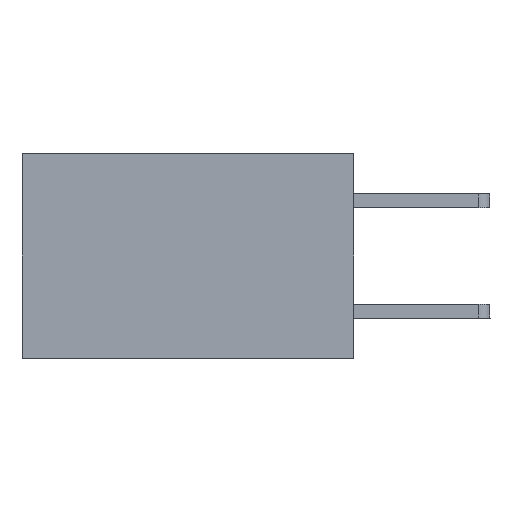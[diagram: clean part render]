
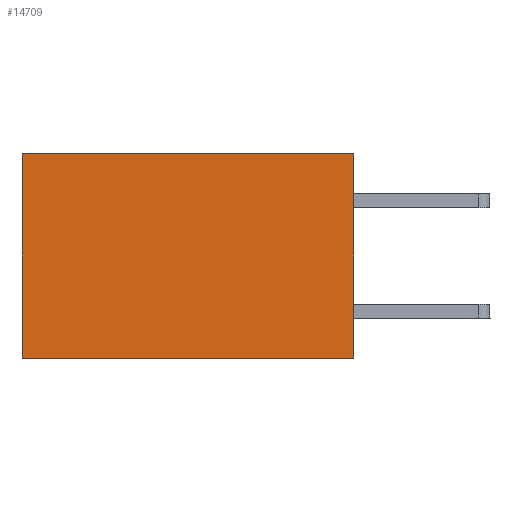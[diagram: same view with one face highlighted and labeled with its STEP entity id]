
A CAD part, left-side view. The second image highlights one B-rep face of the part: STEP entity #14709.
In plain terms, the highlighted planar face has unit normal (-1, 0, 0).
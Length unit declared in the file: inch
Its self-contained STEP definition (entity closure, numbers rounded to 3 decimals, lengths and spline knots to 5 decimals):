
#1321 = CARTESIAN_POINT ( 'NONE',  ( 0.2875, 0., 0. ) ) ;
#1728 = EDGE_CURVE ( 'NONE', #2367, #10280, #5850, .T. ) ;
#1933 = DIRECTION ( 'NONE',  ( 0., 0., -1. ) ) ;
#2138 = LINE ( 'NONE', #5741, #4525 ) ;
#2367 = VERTEX_POINT ( 'NONE', #13669 ) ;
#2877 = VECTOR ( 'NONE', #1933, 39.37008 ) ;
#3353 = DIRECTION ( 'NONE',  ( 0., 1., 0. ) ) ;
#3823 = ORIENTED_EDGE ( 'NONE', *, *, #1728, .F. ) ;
#4215 = LINE ( 'NONE', #5221, #2877 ) ;
#4525 = VECTOR ( 'NONE', #3353, 39.37008 ) ;
#4901 = ORIENTED_EDGE ( 'NONE', *, *, #7709, .T. ) ;
#4930 = PLANE ( 'NONE',  #6812 ) ;
#5221 = CARTESIAN_POINT ( 'NONE',  ( 0.2875, 0.6, 0. ) ) ;
#5741 = CARTESIAN_POINT ( 'NONE',  ( 0.2875, 0., 0. ) ) ;
#5850 = LINE ( 'NONE', #10499, #12642 ) ;
#6453 = CARTESIAN_POINT ( 'NONE',  ( 0.2875, 0., -0.37 ) ) ;
#6812 = AXIS2_PLACEMENT_3D ( 'NONE', #1321, #10638, #8597 ) ;
#6853 = CARTESIAN_POINT ( 'NONE',  ( 0.2875, 0.6, -0.37 ) ) ;
#7210 = EDGE_CURVE ( 'NONE', #11978, #9052, #4215, .T. ) ;
#7233 = EDGE_CURVE ( 'NONE', #10280, #9052, #9878, .T. ) ;
#7252 = EDGE_LOOP ( 'NONE', ( #12729, #7450, #3823, #4901 ) ) ;
#7450 = ORIENTED_EDGE ( 'NONE', *, *, #7233, .F. ) ;
#7600 = DIRECTION ( 'NONE',  ( 0., 1., 0. ) ) ;
#7709 = EDGE_CURVE ( 'NONE', #2367, #11978, #2138, .T. ) ;
#8219 = DIRECTION ( 'NONE',  ( 0., 0., -1. ) ) ;
#8597 = DIRECTION ( 'NONE',  ( 0., 0., -1. ) ) ;
#9052 = VERTEX_POINT ( 'NONE', #6853 ) ;
#9426 = FACE_OUTER_BOUND ( 'NONE', #7252, .T. ) ;
#9721 = VECTOR ( 'NONE', #7600, 39.37008 ) ;
#9878 = LINE ( 'NONE', #6453, #9721 ) ;
#10280 = VERTEX_POINT ( 'NONE', #11043 ) ;
#10499 = CARTESIAN_POINT ( 'NONE',  ( 0.2875, 0., 0. ) ) ;
#10638 = DIRECTION ( 'NONE',  ( 1., 0., 0. ) ) ;
#11043 = CARTESIAN_POINT ( 'NONE',  ( 0.2875, 0., -0.37 ) ) ;
#11978 = VERTEX_POINT ( 'NONE', #12786 ) ;
#12642 = VECTOR ( 'NONE', #8219, 39.37008 ) ;
#12729 = ORIENTED_EDGE ( 'NONE', *, *, #7210, .T. ) ;
#12786 = CARTESIAN_POINT ( 'NONE',  ( 0.2875, 0.6, 0. ) ) ;
#13669 = CARTESIAN_POINT ( 'NONE',  ( 0.2875, 0., 0. ) ) ;
#14709 = ADVANCED_FACE ( 'NONE', ( #9426 ), #4930, .F. ) ;
